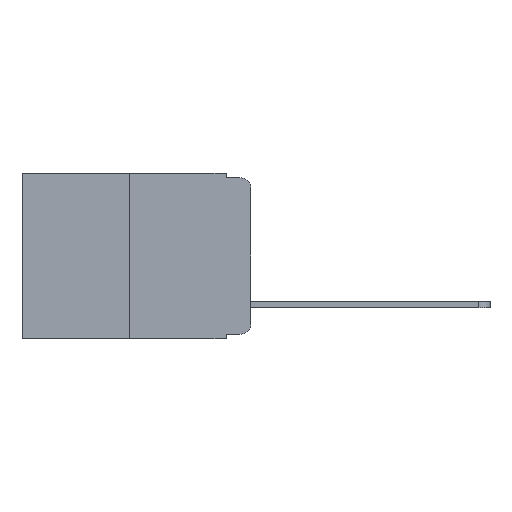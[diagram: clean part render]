
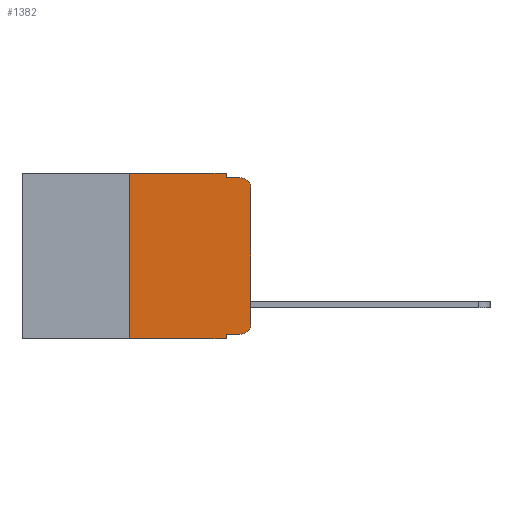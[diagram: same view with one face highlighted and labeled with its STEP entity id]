
A CAD part, left-side view. The second image highlights one B-rep face of the part: STEP entity #1382.
In plain terms, the highlighted planar face has unit normal (-1, 0, 0).
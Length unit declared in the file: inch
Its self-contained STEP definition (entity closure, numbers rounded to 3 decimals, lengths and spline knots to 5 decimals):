
#117 = VECTOR ( 'NONE', #22935, 39.37008 ) ;
#124 = DIRECTION ( 'NONE',  ( -1., 0., 0. ) ) ;
#979 = VERTEX_POINT ( 'NONE', #12053 ) ;
#988 = CARTESIAN_POINT ( 'NONE',  ( 0., 0.051, -0.343 ) ) ;
#1382 = ADVANCED_FACE ( 'NONE', ( #17583 ), #20544, .F. ) ;
#1493 = CARTESIAN_POINT ( 'NONE',  ( 0., 0.02, -0.01 ) ) ;
#1906 = DIRECTION ( 'NONE',  ( 0., 0., -1. ) ) ;
#2007 = CARTESIAN_POINT ( 'NONE',  ( 0., 0., -0.03 ) ) ;
#2056 = ORIENTED_EDGE ( 'NONE', *, *, #21654, .T. ) ;
#2726 = VECTOR ( 'NONE', #12968, 39.37008 ) ;
#3148 = DIRECTION ( 'NONE',  ( 0., -1., 0. ) ) ;
#3298 = VECTOR ( 'NONE', #15081, 39.37008 ) ;
#3340 = ORIENTED_EDGE ( 'NONE', *, *, #12819, .T. ) ;
#4061 = VERTEX_POINT ( 'NONE', #1493 ) ;
#4077 = CARTESIAN_POINT ( 'NONE',  ( 0., 0., 0. ) ) ;
#4872 = VECTOR ( 'NONE', #23055, 39.37008 ) ;
#4979 = CIRCLE ( 'NONE', #7122, 0.02 ) ;
#5053 = AXIS2_PLACEMENT_3D ( 'NONE', #22428, #8085, #8254 ) ;
#5196 = VERTEX_POINT ( 'NONE', #2007 ) ;
#5675 = ORIENTED_EDGE ( 'NONE', *, *, #22374, .T. ) ;
#6077 = EDGE_CURVE ( 'NONE', #8580, #4061, #16451, .T. ) ;
#6413 = VERTEX_POINT ( 'NONE', #21347 ) ;
#6821 = ORIENTED_EDGE ( 'NONE', *, *, #6077, .F. ) ;
#6944 = ORIENTED_EDGE ( 'NONE', *, *, #7890, .F. ) ;
#7122 = AXIS2_PLACEMENT_3D ( 'NONE', #14301, #124, #1906 ) ;
#7533 = EDGE_CURVE ( 'NONE', #15247, #10757, #14684, .T. ) ;
#7639 = CARTESIAN_POINT ( 'NONE',  ( 0., 0.051, -0.333 ) ) ;
#7890 = EDGE_CURVE ( 'NONE', #17773, #8580, #10755, .T. ) ;
#8085 = DIRECTION ( 'NONE',  ( 1., 0., 0. ) ) ;
#8254 = DIRECTION ( 'NONE',  ( 0., 0., -1. ) ) ;
#8378 = VECTOR ( 'NONE', #3148, 39.37008 ) ;
#8533 = ORIENTED_EDGE ( 'NONE', *, *, #7533, .F. ) ;
#8580 = VERTEX_POINT ( 'NONE', #9817 ) ;
#8622 = CARTESIAN_POINT ( 'NONE',  ( 0., 0.25, -0.343 ) ) ;
#9438 = VECTOR ( 'NONE', #22205, 39.37008 ) ;
#9443 = CARTESIAN_POINT ( 'NONE',  ( 0., 0.02, -0.313 ) ) ;
#9532 = CARTESIAN_POINT ( 'NONE',  ( 0., 0.051, -0.01 ) ) ;
#9817 = CARTESIAN_POINT ( 'NONE',  ( 0., 0.051, -0.01 ) ) ;
#9932 = CIRCLE ( 'NONE', #16406, 0.02 ) ;
#10071 = CARTESIAN_POINT ( 'NONE',  ( 0., 0.25, 0. ) ) ;
#10755 = LINE ( 'NONE', #14926, #20568 ) ;
#10757 = VERTEX_POINT ( 'NONE', #988 ) ;
#10787 = LINE ( 'NONE', #10071, #12738 ) ;
#11174 = CARTESIAN_POINT ( 'NONE',  ( 0., 0., -0.313 ) ) ;
#11271 = CARTESIAN_POINT ( 'NONE',  ( 0., 0.051, 0. ) ) ;
#11356 = EDGE_CURVE ( 'NONE', #16113, #6413, #10787, .T. ) ;
#11750 = LINE ( 'NONE', #12887, #2726 ) ;
#12053 = CARTESIAN_POINT ( 'NONE',  ( 0., 0.02, -0.333 ) ) ;
#12738 = VECTOR ( 'NONE', #13645, 39.37008 ) ;
#12819 = EDGE_CURVE ( 'NONE', #979, #13345, #9932, .T. ) ;
#12887 = CARTESIAN_POINT ( 'NONE',  ( 0., 0.473, -0.343 ) ) ;
#12968 = DIRECTION ( 'NONE',  ( 0., -1., 0. ) ) ;
#13014 = LINE ( 'NONE', #14032, #4872 ) ;
#13345 = VERTEX_POINT ( 'NONE', #11174 ) ;
#13645 = DIRECTION ( 'NONE',  ( 0., 0., 1. ) ) ;
#14032 = CARTESIAN_POINT ( 'NONE',  ( 0., 0.473, 0. ) ) ;
#14301 = CARTESIAN_POINT ( 'NONE',  ( 0., 0.02, -0.03 ) ) ;
#14684 = LINE ( 'NONE', #22703, #117 ) ;
#14926 = CARTESIAN_POINT ( 'NONE',  ( 0., 0.051, 0. ) ) ;
#15081 = DIRECTION ( 'NONE',  ( 0., 0., 1. ) ) ;
#15124 = EDGE_CURVE ( 'NONE', #5196, #4061, #4979, .T. ) ;
#15247 = VERTEX_POINT ( 'NONE', #7639 ) ;
#15730 = CARTESIAN_POINT ( 'NONE',  ( 0., 0.051, -0.333 ) ) ;
#16113 = VERTEX_POINT ( 'NONE', #8622 ) ;
#16215 = LINE ( 'NONE', #15730, #8378 ) ;
#16406 = AXIS2_PLACEMENT_3D ( 'NONE', #9443, #16418, #21975 ) ;
#16418 = DIRECTION ( 'NONE',  ( -1., 0., 0. ) ) ;
#16451 = LINE ( 'NONE', #9532, #9438 ) ;
#16722 = DIRECTION ( 'NONE',  ( 0., 0., -1. ) ) ;
#16939 = EDGE_CURVE ( 'NONE', #6413, #17773, #13014, .T. ) ;
#17073 = LINE ( 'NONE', #4077, #3298 ) ;
#17583 = FACE_OUTER_BOUND ( 'NONE', #22614, .T. ) ;
#17773 = VERTEX_POINT ( 'NONE', #11271 ) ;
#20175 = ORIENTED_EDGE ( 'NONE', *, *, #11356, .F. ) ;
#20267 = ORIENTED_EDGE ( 'NONE', *, *, #16939, .F. ) ;
#20316 = ORIENTED_EDGE ( 'NONE', *, *, #15124, .T. ) ;
#20544 = PLANE ( 'NONE',  #5053 ) ;
#20568 = VECTOR ( 'NONE', #16722, 39.37008 ) ;
#21347 = CARTESIAN_POINT ( 'NONE',  ( 0., 0.25, 0. ) ) ;
#21623 = EDGE_CURVE ( 'NONE', #16113, #10757, #11750, .T. ) ;
#21639 = ORIENTED_EDGE ( 'NONE', *, *, #21623, .T. ) ;
#21654 = EDGE_CURVE ( 'NONE', #13345, #5196, #17073, .T. ) ;
#21975 = DIRECTION ( 'NONE',  ( 0., 0., -1. ) ) ;
#22205 = DIRECTION ( 'NONE',  ( 0., -1., 0. ) ) ;
#22374 = EDGE_CURVE ( 'NONE', #15247, #979, #16215, .T. ) ;
#22428 = CARTESIAN_POINT ( 'NONE',  ( 0., 0.473, 0. ) ) ;
#22614 = EDGE_LOOP ( 'NONE', ( #2056, #20316, #6821, #6944, #20267, #20175, #21639, #8533, #5675, #3340 ) ) ;
#22703 = CARTESIAN_POINT ( 'NONE',  ( 0., 0.051, 0. ) ) ;
#22935 = DIRECTION ( 'NONE',  ( 0., 0., -1. ) ) ;
#23055 = DIRECTION ( 'NONE',  ( 0., -1., 0. ) ) ;
